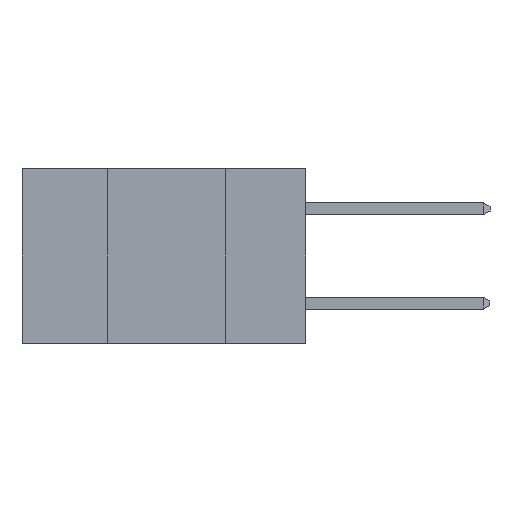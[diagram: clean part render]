
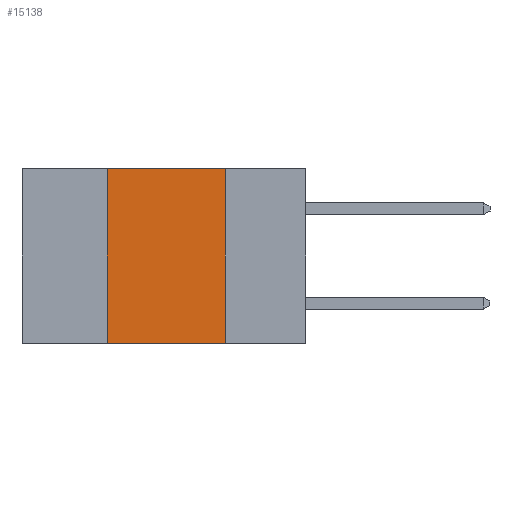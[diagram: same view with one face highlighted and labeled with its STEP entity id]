
A CAD part, left-side view. The second image highlights one B-rep face of the part: STEP entity #15138.
In plain terms, the highlighted planar face has unit normal (-1, 0, 0).
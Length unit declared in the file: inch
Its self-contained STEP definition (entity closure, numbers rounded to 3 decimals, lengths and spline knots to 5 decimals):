
#420 = LINE ( 'NONE', #7490, #3834 ) ;
#883 = CARTESIAN_POINT ( 'NONE',  ( 0., 0.42, 0. ) ) ;
#971 = ORIENTED_EDGE ( 'NONE', *, *, #10853, .T. ) ;
#1700 = CARTESIAN_POINT ( 'NONE',  ( 0., 0.6, 0. ) ) ;
#1907 = CARTESIAN_POINT ( 'NONE',  ( 0., 0.17, 0. ) ) ;
#2495 = DIRECTION ( 'NONE',  ( 0., 0., -1. ) ) ;
#2849 = VECTOR ( 'NONE', #9325, 39.37008 ) ;
#3163 = CARTESIAN_POINT ( 'NONE',  ( 0., 0.42, -0.37 ) ) ;
#3404 = LINE ( 'NONE', #10097, #6052 ) ;
#3834 = VECTOR ( 'NONE', #15777, 39.37008 ) ;
#4180 = EDGE_LOOP ( 'NONE', ( #6527, #13963, #4627, #971 ) ) ;
#4627 = ORIENTED_EDGE ( 'NONE', *, *, #13684, .F. ) ;
#5120 = DIRECTION ( 'NONE',  ( 0., 0., 1. ) ) ;
#6052 = VECTOR ( 'NONE', #5120, 39.37008 ) ;
#6383 = CARTESIAN_POINT ( 'NONE',  ( 0., 0.17, 0. ) ) ;
#6527 = ORIENTED_EDGE ( 'NONE', *, *, #9612, .F. ) ;
#6540 = LINE ( 'NONE', #6383, #12973 ) ;
#6775 = CARTESIAN_POINT ( 'NONE',  ( 0., 0.6, 0. ) ) ;
#6827 = DIRECTION ( 'NONE',  ( 1., 0., 0. ) ) ;
#7490 = CARTESIAN_POINT ( 'NONE',  ( 0., 0.6, -0.37 ) ) ;
#8257 = CARTESIAN_POINT ( 'NONE',  ( 0., 0.17, -0.37 ) ) ;
#8567 = VERTEX_POINT ( 'NONE', #883 ) ;
#9075 = FACE_OUTER_BOUND ( 'NONE', #4180, .T. ) ;
#9261 = VERTEX_POINT ( 'NONE', #3163 ) ;
#9325 = DIRECTION ( 'NONE',  ( 0., -1., 0. ) ) ;
#9612 = EDGE_CURVE ( 'NONE', #13973, #14481, #6540, .T. ) ;
#10097 = CARTESIAN_POINT ( 'NONE',  ( 0., 0.42, 0. ) ) ;
#10853 = EDGE_CURVE ( 'NONE', #9261, #14481, #420, .T. ) ;
#11618 = PLANE ( 'NONE',  #12156 ) ;
#12156 = AXIS2_PLACEMENT_3D ( 'NONE', #6775, #6827, #15163 ) ;
#12610 = EDGE_CURVE ( 'NONE', #8567, #13973, #15801, .T. ) ;
#12973 = VECTOR ( 'NONE', #2495, 39.37008 ) ;
#13684 = EDGE_CURVE ( 'NONE', #9261, #8567, #3404, .T. ) ;
#13963 = ORIENTED_EDGE ( 'NONE', *, *, #12610, .F. ) ;
#13973 = VERTEX_POINT ( 'NONE', #1907 ) ;
#14481 = VERTEX_POINT ( 'NONE', #8257 ) ;
#15138 = ADVANCED_FACE ( 'NONE', ( #9075 ), #11618, .F. ) ;
#15163 = DIRECTION ( 'NONE',  ( 0., 0., -1. ) ) ;
#15777 = DIRECTION ( 'NONE',  ( 0., -1., 0. ) ) ;
#15801 = LINE ( 'NONE', #1700, #2849 ) ;
